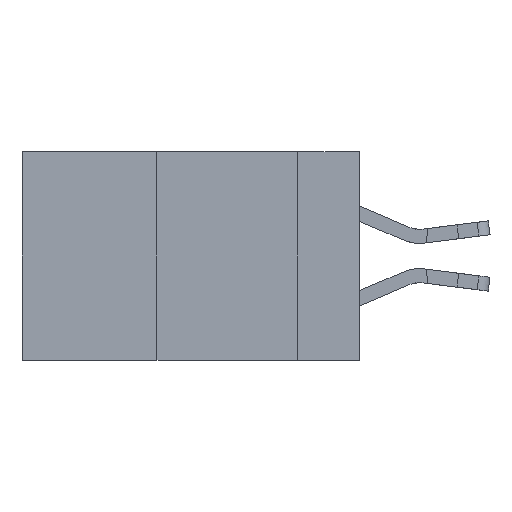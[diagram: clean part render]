
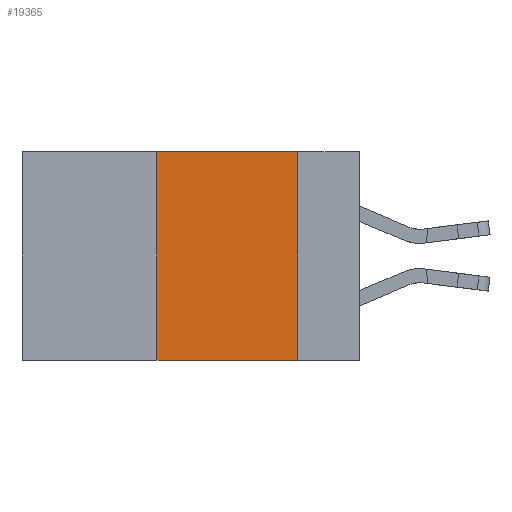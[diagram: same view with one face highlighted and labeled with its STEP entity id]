
A CAD part, left-side view. The second image highlights one B-rep face of the part: STEP entity #19365.
In plain terms, the highlighted planar face has unit normal (-1, 0, 0).
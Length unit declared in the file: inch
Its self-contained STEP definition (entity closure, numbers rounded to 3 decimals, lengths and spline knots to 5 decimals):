
#558 = LINE ( 'NONE', #5460, #12262 ) ;
#2069 = CARTESIAN_POINT ( 'NONE',  ( 0., 0.36, 0. ) ) ;
#2176 = VERTEX_POINT ( 'NONE', #14286 ) ;
#2742 = DIRECTION ( 'NONE',  ( 0., -1., 0. ) ) ;
#3531 = ORIENTED_EDGE ( 'NONE', *, *, #18357, .F. ) ;
#3570 = VECTOR ( 'NONE', #2742, 39.37008 ) ;
#3735 = VECTOR ( 'NONE', #11528, 39.37008 ) ;
#3751 = VERTEX_POINT ( 'NONE', #19300 ) ;
#4164 = VERTEX_POINT ( 'NONE', #5624 ) ;
#5254 = EDGE_CURVE ( 'NONE', #4164, #3751, #20922, .T. ) ;
#5460 = CARTESIAN_POINT ( 'NONE',  ( 0., 0.11, 0. ) ) ;
#5624 = CARTESIAN_POINT ( 'NONE',  ( 0., 0.36, -0.37 ) ) ;
#6084 = LINE ( 'NONE', #21929, #22683 ) ;
#6935 = VERTEX_POINT ( 'NONE', #2069 ) ;
#7078 = CARTESIAN_POINT ( 'NONE',  ( 0., 0.6, -0.37 ) ) ;
#7667 = DIRECTION ( 'NONE',  ( 0., 0., -1. ) ) ;
#8206 = EDGE_CURVE ( 'NONE', #4164, #6935, #21084, .T. ) ;
#9137 = CARTESIAN_POINT ( 'NONE',  ( 0., 0.6, 0. ) ) ;
#9306 = CARTESIAN_POINT ( 'NONE',  ( 0., 0.36, 0. ) ) ;
#11208 = DIRECTION ( 'NONE',  ( 0., -1., 0. ) ) ;
#11346 = DIRECTION ( 'NONE',  ( 1., 0., 0. ) ) ;
#11528 = DIRECTION ( 'NONE',  ( 0., 0., 1. ) ) ;
#12262 = VECTOR ( 'NONE', #7667, 39.37008 ) ;
#14286 = CARTESIAN_POINT ( 'NONE',  ( 0., 0.11, 0. ) ) ;
#15432 = AXIS2_PLACEMENT_3D ( 'NONE', #9137, #11346, #26390 ) ;
#15498 = EDGE_CURVE ( 'NONE', #6935, #2176, #6084, .T. ) ;
#16860 = EDGE_LOOP ( 'NONE', ( #3531, #21545, #18533, #25592 ) ) ;
#18357 = EDGE_CURVE ( 'NONE', #2176, #3751, #558, .T. ) ;
#18533 = ORIENTED_EDGE ( 'NONE', *, *, #8206, .F. ) ;
#19300 = CARTESIAN_POINT ( 'NONE',  ( 0., 0.11, -0.37 ) ) ;
#19365 = ADVANCED_FACE ( 'NONE', ( #24648 ), #22067, .F. ) ;
#20922 = LINE ( 'NONE', #7078, #3570 ) ;
#21084 = LINE ( 'NONE', #9306, #3735 ) ;
#21545 = ORIENTED_EDGE ( 'NONE', *, *, #15498, .F. ) ;
#21929 = CARTESIAN_POINT ( 'NONE',  ( 0., 0.6, 0. ) ) ;
#22067 = PLANE ( 'NONE',  #15432 ) ;
#22683 = VECTOR ( 'NONE', #11208, 39.37008 ) ;
#24648 = FACE_OUTER_BOUND ( 'NONE', #16860, .T. ) ;
#25592 = ORIENTED_EDGE ( 'NONE', *, *, #5254, .T. ) ;
#26390 = DIRECTION ( 'NONE',  ( 0., 0., -1. ) ) ;
